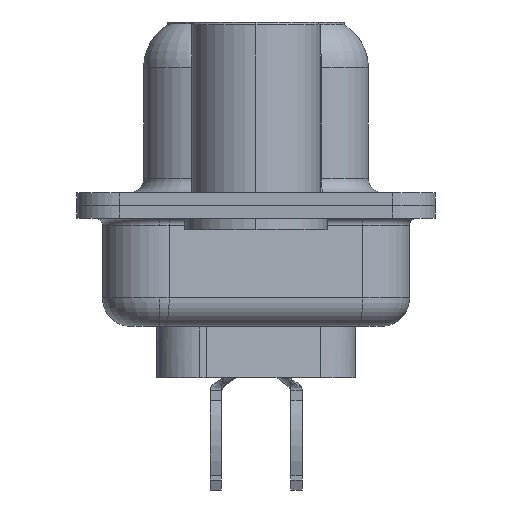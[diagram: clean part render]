
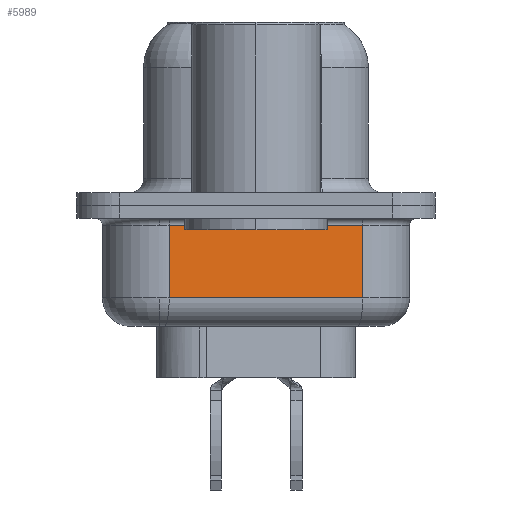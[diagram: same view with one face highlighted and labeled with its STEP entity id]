
A CAD part, left-side view. The second image highlights one B-rep face of the part: STEP entity #5989.
In plain terms, the highlighted planar face has unit normal (-0.985, -0.174, 0).
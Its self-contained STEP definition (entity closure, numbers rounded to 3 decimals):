
#180 = VECTOR ( 'NONE', #10837, 1000. ) ;
#222 = EDGE_CURVE ( 'NONE', #2254, #18988, #7337, .T. ) ;
#1027 = PLANE ( 'NONE',  #11159 ) ;
#2237 = VECTOR ( 'NONE', #13738, 1000. ) ;
#2254 = VERTEX_POINT ( 'NONE', #2677 ) ;
#2615 = DIRECTION ( 'NONE',  ( -0.174, 0.985, 0. ) ) ;
#2677 = CARTESIAN_POINT ( 'NONE',  ( 4.074, -3.747, -0.7 ) ) ;
#5323 = EDGE_CURVE ( 'NONE', #20697, #15642, #8372, .T. ) ;
#5989 = ADVANCED_FACE ( 'NONE', ( #6080 ), #1027, .F. ) ;
#5999 = CARTESIAN_POINT ( 'NONE',  ( 4.074, -3.747, -4.25 ) ) ;
#6080 = FACE_OUTER_BOUND ( 'NONE', #18693, .T. ) ;
#6103 = DIRECTION ( 'NONE',  ( 0., 0., 1. ) ) ;
#7337 = LINE ( 'NONE', #19950, #2237 ) ;
#8372 = LINE ( 'NONE', #13089, #13827 ) ;
#10837 = DIRECTION ( 'NONE',  ( 0., 0., 1. ) ) ;
#11159 = AXIS2_PLACEMENT_3D ( 'NONE', #18724, #12311, #2615 ) ;
#12146 = ORIENTED_EDGE ( 'NONE', *, *, #5323, .T. ) ;
#12311 = DIRECTION ( 'NONE',  ( 0.985, 0.174, 0. ) ) ;
#12642 = CARTESIAN_POINT ( 'NONE',  ( 4.074, -3.747, -3.25 ) ) ;
#13004 = CARTESIAN_POINT ( 'NONE',  ( 2.875, 3.053, -0.7 ) ) ;
#13089 = CARTESIAN_POINT ( 'NONE',  ( 2.875, 3.053, -3.25 ) ) ;
#13195 = DIRECTION ( 'NONE',  ( 0.174, -0.985, 0. ) ) ;
#13362 = CARTESIAN_POINT ( 'NONE',  ( 2.875, 3.053, -3.25 ) ) ;
#13738 = DIRECTION ( 'NONE',  ( -0.174, 0.985, 0. ) ) ;
#13827 = VECTOR ( 'NONE', #13195, 1000. ) ;
#14215 = VECTOR ( 'NONE', #6103, 1000. ) ;
#15063 = ORIENTED_EDGE ( 'NONE', *, *, #222, .T. ) ;
#15127 = EDGE_CURVE ( 'NONE', #15642, #2254, #18744, .T. ) ;
#15580 = CARTESIAN_POINT ( 'NONE',  ( 2.875, 3.053, -4.25 ) ) ;
#15642 = VERTEX_POINT ( 'NONE', #12642 ) ;
#17816 = EDGE_CURVE ( 'NONE', #20697, #18988, #18934, .T. ) ;
#18693 = EDGE_LOOP ( 'NONE', ( #20055, #12146, #20173, #15063 ) ) ;
#18724 = CARTESIAN_POINT ( 'NONE',  ( 2.875, 3.053, -4.25 ) ) ;
#18744 = LINE ( 'NONE', #5999, #14215 ) ;
#18934 = LINE ( 'NONE', #15580, #180 ) ;
#18988 = VERTEX_POINT ( 'NONE', #13004 ) ;
#19950 = CARTESIAN_POINT ( 'NONE',  ( 2.875, 3.053, -0.7 ) ) ;
#20055 = ORIENTED_EDGE ( 'NONE', *, *, #17816, .F. ) ;
#20173 = ORIENTED_EDGE ( 'NONE', *, *, #15127, .T. ) ;
#20697 = VERTEX_POINT ( 'NONE', #13362 ) ;
